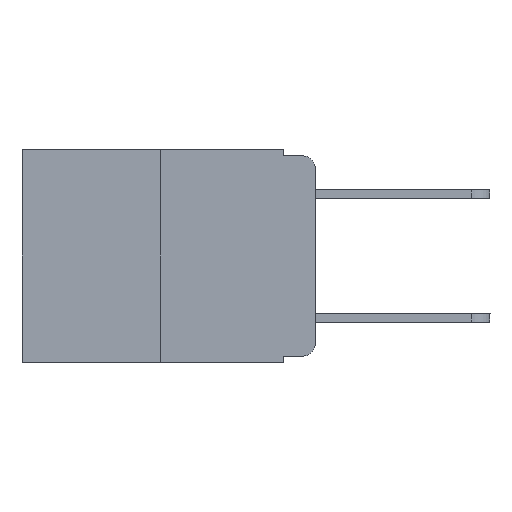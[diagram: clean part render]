
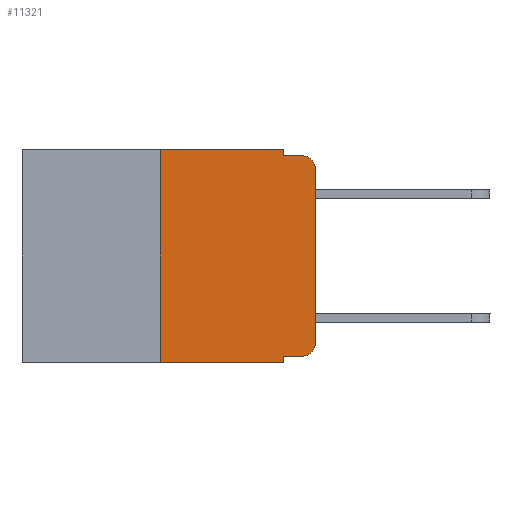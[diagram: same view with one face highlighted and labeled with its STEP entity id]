
A CAD part, left-side view. The second image highlights one B-rep face of the part: STEP entity #11321.
In plain terms, the highlighted planar face has unit normal (-1, 0, 0).
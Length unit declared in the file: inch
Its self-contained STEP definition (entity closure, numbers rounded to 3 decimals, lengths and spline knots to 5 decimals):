
#362 = EDGE_CURVE ( 'NONE', #16341, #11507, #22708, .T. ) ;
#451 = DIRECTION ( 'NONE',  ( 0., 0., 1. ) ) ;
#609 = EDGE_CURVE ( 'NONE', #3478, #16341, #12343, .T. ) ;
#743 = CIRCLE ( 'NONE', #13687, 0.02 ) ;
#1147 = AXIS2_PLACEMENT_3D ( 'NONE', #6850, #21370, #19777 ) ;
#1180 = EDGE_CURVE ( 'NONE', #16104, #22577, #20915, .T. ) ;
#1225 = VERTEX_POINT ( 'NONE', #17332 ) ;
#1654 = CARTESIAN_POINT ( 'NONE',  ( 0., 0.473, -0.343 ) ) ;
#1891 = EDGE_CURVE ( 'NONE', #3478, #5429, #22663, .T. ) ;
#2357 = EDGE_CURVE ( 'NONE', #13027, #5429, #19762, .T. ) ;
#2569 = CARTESIAN_POINT ( 'NONE',  ( 0., 0., 0. ) ) ;
#2889 = CARTESIAN_POINT ( 'NONE',  ( 0., 0.02, -0.313 ) ) ;
#2965 = ORIENTED_EDGE ( 'NONE', *, *, #7591, .F. ) ;
#3478 = VERTEX_POINT ( 'NONE', #8055 ) ;
#3491 = VECTOR ( 'NONE', #3879, 39.37008 ) ;
#3642 = DIRECTION ( 'NONE',  ( 0., -1., 0. ) ) ;
#3879 = DIRECTION ( 'NONE',  ( 0., -1., 0. ) ) ;
#5429 = VERTEX_POINT ( 'NONE', #22101 ) ;
#6027 = VECTOR ( 'NONE', #451, 39.37008 ) ;
#6850 = CARTESIAN_POINT ( 'NONE',  ( 0., 0.473, 0. ) ) ;
#7591 = EDGE_CURVE ( 'NONE', #22577, #10197, #9173, .T. ) ;
#7793 = ORIENTED_EDGE ( 'NONE', *, *, #20797, .F. ) ;
#8055 = CARTESIAN_POINT ( 'NONE',  ( 0., 0.051, -0.333 ) ) ;
#8091 = DIRECTION ( 'NONE',  ( 0., 0., -1. ) ) ;
#8363 = DIRECTION ( 'NONE',  ( 0., -1., 0. ) ) ;
#8794 = DIRECTION ( 'NONE',  ( 0., -1., 0. ) ) ;
#9173 = LINE ( 'NONE', #18211, #11217 ) ;
#10197 = VERTEX_POINT ( 'NONE', #15537 ) ;
#11197 = CARTESIAN_POINT ( 'NONE',  ( 0., 0.051, 0. ) ) ;
#11217 = VECTOR ( 'NONE', #3642, 39.37008 ) ;
#11321 = ADVANCED_FACE ( 'NONE', ( #21669 ), #19611, .F. ) ;
#11507 = VERTEX_POINT ( 'NONE', #20404 ) ;
#11596 = CARTESIAN_POINT ( 'NONE',  ( 0., 0.02, -0.333 ) ) ;
#12094 = ORIENTED_EDGE ( 'NONE', *, *, #1891, .F. ) ;
#12343 = LINE ( 'NONE', #15114, #18390 ) ;
#12454 = ORIENTED_EDGE ( 'NONE', *, *, #1180, .F. ) ;
#12681 = AXIS2_PLACEMENT_3D ( 'NONE', #2889, #20116, #16851 ) ;
#12813 = LINE ( 'NONE', #14915, #22859 ) ;
#13027 = VERTEX_POINT ( 'NONE', #23248 ) ;
#13687 = AXIS2_PLACEMENT_3D ( 'NONE', #21023, #13814, #21106 ) ;
#13814 = DIRECTION ( 'NONE',  ( -1., 0., 0. ) ) ;
#14062 = EDGE_LOOP ( 'NONE', ( #23803, #19596, #2965, #12454, #19021, #7793, #14966, #12094, #16508, #15360 ) ) ;
#14289 = CARTESIAN_POINT ( 'NONE',  ( 0., 0.25, 0. ) ) ;
#14322 = VECTOR ( 'NONE', #15523, 39.37008 ) ;
#14389 = EDGE_CURVE ( 'NONE', #11507, #1225, #18194, .T. ) ;
#14915 = CARTESIAN_POINT ( 'NONE',  ( 0., 0.25, 0. ) ) ;
#14966 = ORIENTED_EDGE ( 'NONE', *, *, #2357, .T. ) ;
#15059 = CARTESIAN_POINT ( 'NONE',  ( 0., 0.473, 0. ) ) ;
#15114 = CARTESIAN_POINT ( 'NONE',  ( 0., 0.051, -0.333 ) ) ;
#15143 = DIRECTION ( 'NONE',  ( 0., 0., 1. ) ) ;
#15360 = ORIENTED_EDGE ( 'NONE', *, *, #362, .T. ) ;
#15523 = DIRECTION ( 'NONE',  ( 0., 0., -1. ) ) ;
#15537 = CARTESIAN_POINT ( 'NONE',  ( 0., 0.02, -0.01 ) ) ;
#16104 = VERTEX_POINT ( 'NONE', #11197 ) ;
#16341 = VERTEX_POINT ( 'NONE', #11596 ) ;
#16508 = ORIENTED_EDGE ( 'NONE', *, *, #609, .T. ) ;
#16851 = DIRECTION ( 'NONE',  ( 0., 0., -1. ) ) ;
#17332 = CARTESIAN_POINT ( 'NONE',  ( 0., 0., -0.03 ) ) ;
#18194 = LINE ( 'NONE', #2569, #6027 ) ;
#18211 = CARTESIAN_POINT ( 'NONE',  ( 0., 0.051, -0.01 ) ) ;
#18390 = VECTOR ( 'NONE', #8363, 39.37008 ) ;
#18911 = VECTOR ( 'NONE', #8794, 39.37008 ) ;
#18933 = VERTEX_POINT ( 'NONE', #14289 ) ;
#19021 = ORIENTED_EDGE ( 'NONE', *, *, #20907, .F. ) ;
#19173 = CARTESIAN_POINT ( 'NONE',  ( 0., 0.051, 0. ) ) ;
#19596 = ORIENTED_EDGE ( 'NONE', *, *, #23686, .T. ) ;
#19611 = PLANE ( 'NONE',  #1147 ) ;
#19762 = LINE ( 'NONE', #1654, #18911 ) ;
#19777 = DIRECTION ( 'NONE',  ( 0., 0., -1. ) ) ;
#19975 = LINE ( 'NONE', #15059, #3491 ) ;
#20116 = DIRECTION ( 'NONE',  ( -1., 0., 0. ) ) ;
#20404 = CARTESIAN_POINT ( 'NONE',  ( 0., 0., -0.313 ) ) ;
#20797 = EDGE_CURVE ( 'NONE', #13027, #18933, #12813, .T. ) ;
#20907 = EDGE_CURVE ( 'NONE', #18933, #16104, #19975, .T. ) ;
#20915 = LINE ( 'NONE', #19173, #22693 ) ;
#21023 = CARTESIAN_POINT ( 'NONE',  ( 0., 0.02, -0.03 ) ) ;
#21106 = DIRECTION ( 'NONE',  ( 0., 0., -1. ) ) ;
#21210 = CARTESIAN_POINT ( 'NONE',  ( 0., 0.051, 0. ) ) ;
#21370 = DIRECTION ( 'NONE',  ( 1., 0., 0. ) ) ;
#21669 = FACE_OUTER_BOUND ( 'NONE', #14062, .T. ) ;
#22101 = CARTESIAN_POINT ( 'NONE',  ( 0., 0.051, -0.343 ) ) ;
#22146 = CARTESIAN_POINT ( 'NONE',  ( 0., 0.051, -0.01 ) ) ;
#22577 = VERTEX_POINT ( 'NONE', #22146 ) ;
#22663 = LINE ( 'NONE', #21210, #14322 ) ;
#22693 = VECTOR ( 'NONE', #8091, 39.37008 ) ;
#22708 = CIRCLE ( 'NONE', #12681, 0.02 ) ;
#22859 = VECTOR ( 'NONE', #15143, 39.37008 ) ;
#23248 = CARTESIAN_POINT ( 'NONE',  ( 0., 0.25, -0.343 ) ) ;
#23686 = EDGE_CURVE ( 'NONE', #1225, #10197, #743, .T. ) ;
#23803 = ORIENTED_EDGE ( 'NONE', *, *, #14389, .T. ) ;
